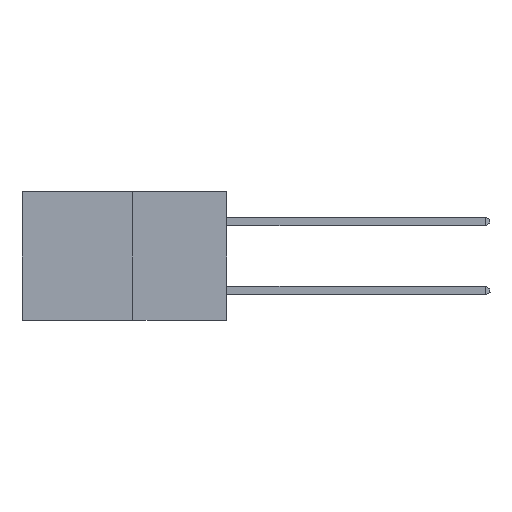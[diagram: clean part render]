
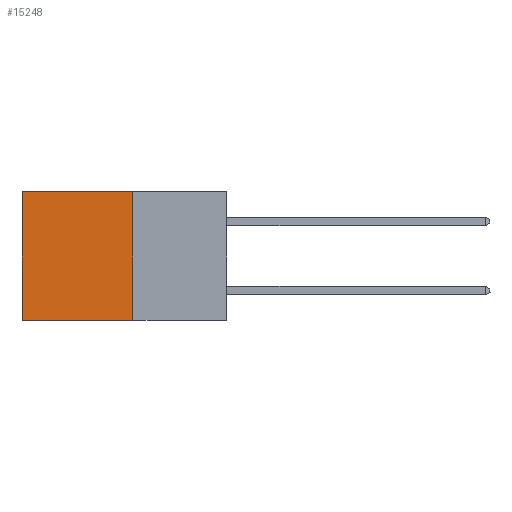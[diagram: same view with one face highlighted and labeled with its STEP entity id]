
A CAD part, left-side view. The second image highlights one B-rep face of the part: STEP entity #15248.
In plain terms, the highlighted planar face has unit normal (-1, 0, 0).
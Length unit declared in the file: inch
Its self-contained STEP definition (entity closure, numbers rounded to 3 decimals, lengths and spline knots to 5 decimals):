
#499 = LINE ( 'NONE', #13759, #23883 ) ;
#664 = VECTOR ( 'NONE', #27666, 39.37008 ) ;
#2586 = VERTEX_POINT ( 'NONE', #11520 ) ;
#3567 = DIRECTION ( 'NONE',  ( 0., 1., 0. ) ) ;
#4069 = ORIENTED_EDGE ( 'NONE', *, *, #21576, .F. ) ;
#5346 = VERTEX_POINT ( 'NONE', #24640 ) ;
#6997 = CARTESIAN_POINT ( 'NONE',  ( 0.277, 0.27, -0.37 ) ) ;
#7171 = DIRECTION ( 'NONE',  ( 0., 1., 0. ) ) ;
#8646 = ORIENTED_EDGE ( 'NONE', *, *, #14875, .F. ) ;
#9022 = VERTEX_POINT ( 'NONE', #11341 ) ;
#9174 = DIRECTION ( 'NONE',  ( 0., 0., -1. ) ) ;
#9641 = LINE ( 'NONE', #16694, #25847 ) ;
#10039 = VERTEX_POINT ( 'NONE', #13546 ) ;
#10965 = ORIENTED_EDGE ( 'NONE', *, *, #26480, .T. ) ;
#11341 = CARTESIAN_POINT ( 'NONE',  ( 0.277, 0.27, -0.37 ) ) ;
#11520 = CARTESIAN_POINT ( 'NONE',  ( 0.277, 0.27, 0. ) ) ;
#11607 = CARTESIAN_POINT ( 'NONE',  ( 0.277, 0.27, -0.37 ) ) ;
#13546 = CARTESIAN_POINT ( 'NONE',  ( 0.277, 0.59, 0. ) ) ;
#13759 = CARTESIAN_POINT ( 'NONE',  ( 0.277, 0.27, 0. ) ) ;
#13840 = EDGE_LOOP ( 'NONE', ( #14574, #8646, #4069, #10965 ) ) ;
#14574 = ORIENTED_EDGE ( 'NONE', *, *, #23053, .T. ) ;
#14875 = EDGE_CURVE ( 'NONE', #9022, #5346, #9641, .T. ) ;
#15248 = ADVANCED_FACE ( 'NONE', ( #27875 ), #20153, .F. ) ;
#16674 = CARTESIAN_POINT ( 'NONE',  ( 0.277, 0.59, -0.37 ) ) ;
#16694 = CARTESIAN_POINT ( 'NONE',  ( 0.277, 0.27, -0.37 ) ) ;
#20153 = PLANE ( 'NONE',  #27425 ) ;
#21576 = EDGE_CURVE ( 'NONE', #2586, #9022, #26869, .T. ) ;
#21704 = VECTOR ( 'NONE', #27005, 39.37008 ) ;
#22354 = DIRECTION ( 'NONE',  ( 1., 0., 0. ) ) ;
#23053 = EDGE_CURVE ( 'NONE', #10039, #5346, #24037, .T. ) ;
#23883 = VECTOR ( 'NONE', #7171, 39.37008 ) ;
#24037 = LINE ( 'NONE', #16674, #664 ) ;
#24640 = CARTESIAN_POINT ( 'NONE',  ( 0.277, 0.59, -0.37 ) ) ;
#25847 = VECTOR ( 'NONE', #3567, 39.37008 ) ;
#26480 = EDGE_CURVE ( 'NONE', #2586, #10039, #499, .T. ) ;
#26869 = LINE ( 'NONE', #11607, #21704 ) ;
#27005 = DIRECTION ( 'NONE',  ( 0., 0., -1. ) ) ;
#27425 = AXIS2_PLACEMENT_3D ( 'NONE', #6997, #22354, #9174 ) ;
#27666 = DIRECTION ( 'NONE',  ( 0., 0., -1. ) ) ;
#27875 = FACE_OUTER_BOUND ( 'NONE', #13840, .T. ) ;
